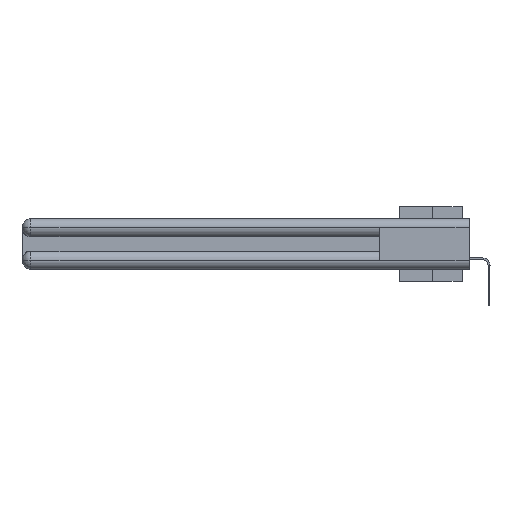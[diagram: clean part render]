
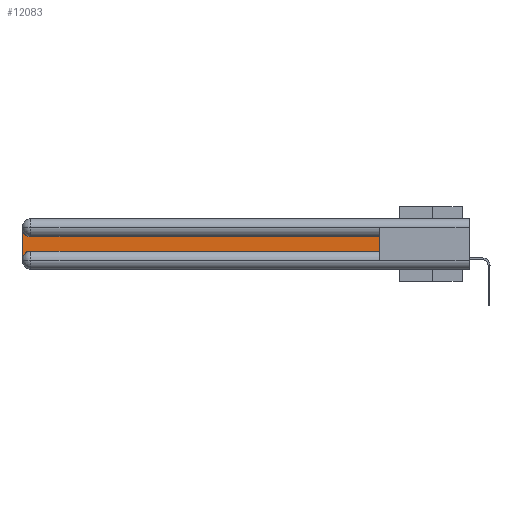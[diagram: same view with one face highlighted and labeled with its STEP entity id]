
A CAD part, left-side view. The second image highlights one B-rep face of the part: STEP entity #12083.
In plain terms, the highlighted planar face has unit normal (-1, 0, 0).
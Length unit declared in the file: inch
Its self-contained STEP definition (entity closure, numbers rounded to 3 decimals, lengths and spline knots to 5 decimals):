
#250 = EDGE_CURVE ( 'NONE', #26192, #18823, #29348, .T. ) ;
#327 = VERTEX_POINT ( 'NONE', #27570 ) ;
#2492 = CIRCLE ( 'NONE', #28620, 0.06 ) ;
#3397 = CARTESIAN_POINT ( 'NONE',  ( 0.075, 0.6, -0.2175 ) ) ;
#6564 = FACE_OUTER_BOUND ( 'NONE', #26226, .T. ) ;
#6931 = CARTESIAN_POINT ( 'NONE',  ( 0.075, 0.6, -0.1225 ) ) ;
#6997 = CARTESIAN_POINT ( 'NONE',  ( 0.075, 2.94, -0.1225 ) ) ;
#7849 = CARTESIAN_POINT ( 'NONE',  ( 0.075, 3., -0.2175 ) ) ;
#8149 = DIRECTION ( 'NONE',  ( 0., 0., -1. ) ) ;
#8765 = EDGE_CURVE ( 'NONE', #18823, #10445, #32866, .T. ) ;
#10445 = VERTEX_POINT ( 'NONE', #19655 ) ;
#10493 = ORIENTED_EDGE ( 'NONE', *, *, #39338, .T. ) ;
#10786 = DIRECTION ( 'NONE',  ( 1., 0., 0. ) ) ;
#12083 = ADVANCED_FACE ( 'NONE', ( #6564 ), #30309, .F. ) ;
#12181 = ORIENTED_EDGE ( 'NONE', *, *, #15033, .T. ) ;
#12760 = DIRECTION ( 'NONE',  ( 0., 1., 0. ) ) ;
#15033 = EDGE_CURVE ( 'NONE', #25148, #327, #26741, .T. ) ;
#15558 = CARTESIAN_POINT ( 'NONE',  ( 0.075, 0.6, -0.2175 ) ) ;
#16229 = CARTESIAN_POINT ( 'NONE',  ( 0.075, 3., -0.2775 ) ) ;
#16423 = DIRECTION ( 'NONE',  ( 0., 0., -1. ) ) ;
#16448 = LINE ( 'NONE', #6931, #20251 ) ;
#16561 = DIRECTION ( 'NONE',  ( 1., 0., 0. ) ) ;
#17345 = CARTESIAN_POINT ( 'NONE',  ( 0.075, 2.94, -0.0625 ) ) ;
#17651 = DIRECTION ( 'NONE',  ( 1., 0., 0. ) ) ;
#18823 = VERTEX_POINT ( 'NONE', #16229 ) ;
#19655 = CARTESIAN_POINT ( 'NONE',  ( 0.075, 2.94, -0.2175 ) ) ;
#20191 = CARTESIAN_POINT ( 'NONE',  ( 0.075, 2.94, -0.2775 ) ) ;
#20251 = VECTOR ( 'NONE', #12760, 39.37008 ) ;
#21221 = VECTOR ( 'NONE', #37888, 39.37008 ) ;
#21241 = AXIS2_PLACEMENT_3D ( 'NONE', #32874, #17651, #23806 ) ;
#22437 = LINE ( 'NONE', #3397, #38675 ) ;
#23433 = VERTEX_POINT ( 'NONE', #6997 ) ;
#23806 = DIRECTION ( 'NONE',  ( 0., 0., -1. ) ) ;
#25148 = VERTEX_POINT ( 'NONE', #15558 ) ;
#25560 = ORIENTED_EDGE ( 'NONE', *, *, #38993, .T. ) ;
#25853 = ORIENTED_EDGE ( 'NONE', *, *, #30508, .T. ) ;
#26192 = VERTEX_POINT ( 'NONE', #36297 ) ;
#26226 = EDGE_LOOP ( 'NONE', ( #25853, #25560, #36940, #27364, #10493, #12181 ) ) ;
#26741 = LINE ( 'NONE', #27962, #33449 ) ;
#27364 = ORIENTED_EDGE ( 'NONE', *, *, #8765, .T. ) ;
#27570 = CARTESIAN_POINT ( 'NONE',  ( 0.075, 0.6, -0.1225 ) ) ;
#27962 = CARTESIAN_POINT ( 'NONE',  ( 0.075, 0.6, -0.2175 ) ) ;
#28620 = AXIS2_PLACEMENT_3D ( 'NONE', #17345, #16561, #16423 ) ;
#29348 = LINE ( 'NONE', #7849, #21221 ) ;
#30309 = PLANE ( 'NONE',  #21241 ) ;
#30508 = EDGE_CURVE ( 'NONE', #327, #23433, #16448, .T. ) ;
#32866 = CIRCLE ( 'NONE', #36212, 0.06 ) ;
#32874 = CARTESIAN_POINT ( 'NONE',  ( 0.075, 3., -0.1225 ) ) ;
#33449 = VECTOR ( 'NONE', #33837, 39.37008 ) ;
#33837 = DIRECTION ( 'NONE',  ( 0., 0., 1. ) ) ;
#33896 = DIRECTION ( 'NONE',  ( 0., -1., 0. ) ) ;
#36212 = AXIS2_PLACEMENT_3D ( 'NONE', #20191, #10786, #8149 ) ;
#36297 = CARTESIAN_POINT ( 'NONE',  ( 0.075, 3., -0.0625 ) ) ;
#36940 = ORIENTED_EDGE ( 'NONE', *, *, #250, .T. ) ;
#37888 = DIRECTION ( 'NONE',  ( 0., 0., -1. ) ) ;
#38675 = VECTOR ( 'NONE', #33896, 39.37008 ) ;
#38993 = EDGE_CURVE ( 'NONE', #23433, #26192, #2492, .T. ) ;
#39338 = EDGE_CURVE ( 'NONE', #10445, #25148, #22437, .T. ) ;
